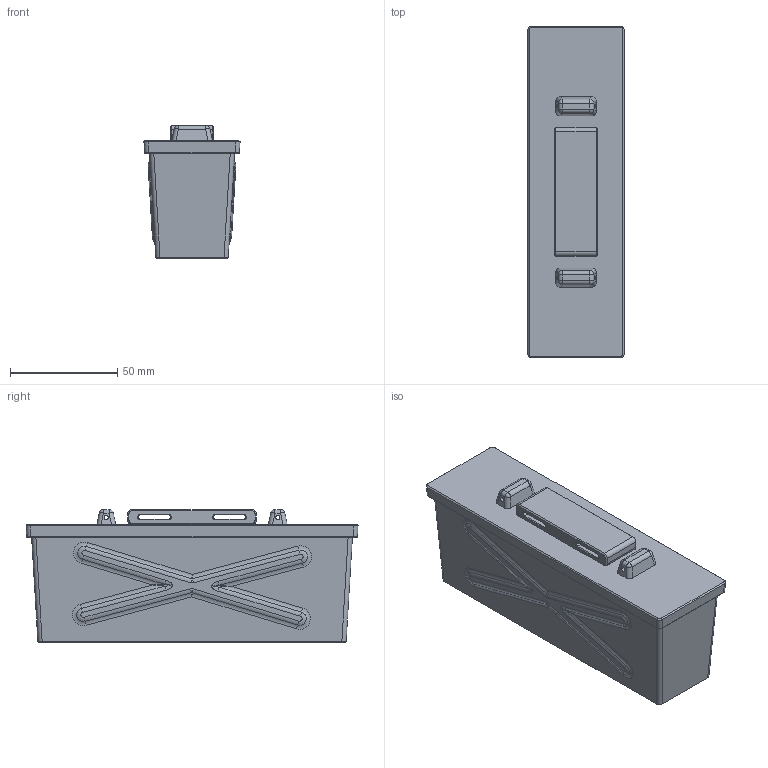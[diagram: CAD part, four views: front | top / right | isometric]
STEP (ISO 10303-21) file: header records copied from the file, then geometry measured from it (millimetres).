
FILE_DESCRIPTION(/* description */ (''),/* implementation_level */ '2;1');
FILE_NAME(/* name */ '22lr 100rd ammo can.stp',/* time_stamp */ '2021-07-17T13:31:35+02:00',/* author */ (''),/* organization */ (''),/* preprocessor_version */ 'ST-DEVELOPER v15.2',/* originating_system */ 'Autodesk Translator Framework v2.0.0.5431',/* authorisation */ '');
FILE_SCHEMA (('AUTOMOTIVE_DESIGN { 1 0 10303 214 3 1 1 }'));
Length unit declared in the file: centimetre
Products named in the file (1): ammo tin v5
Bounding box: 44.9 x 154.9 x 62 mm (x, y, z)
Volume: 94729 mm3; surface area: 70170.9 mm2
Topology: 5 solids, 5 shells, 297 faces, 690 edges, 396 vertices
Faces by surface type: cylinder 110, plane 83, bspline 68, cone 16, sphere 12, torus 8
Full cylindrical faces by diameter (mm): 2 x2
Entity records: 9566 total; most frequent: CARTESIAN_POINT 3024, ORIENTED_EDGE 1352, DIRECTION 1340, EDGE_CURVE 676, AXIS2_PLACEMENT_3D 498, VERTEX_POINT 396, LINE 344, VECTOR 344
